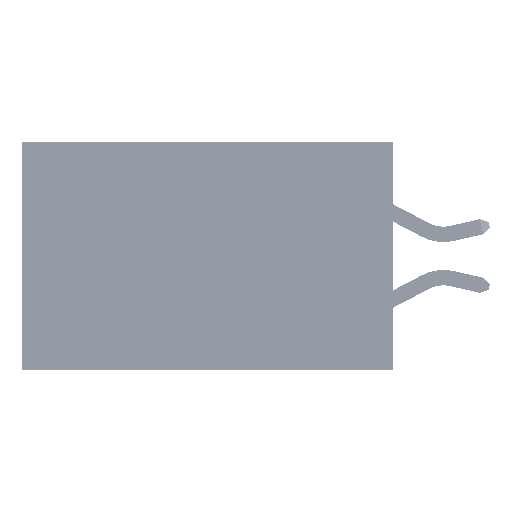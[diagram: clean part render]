
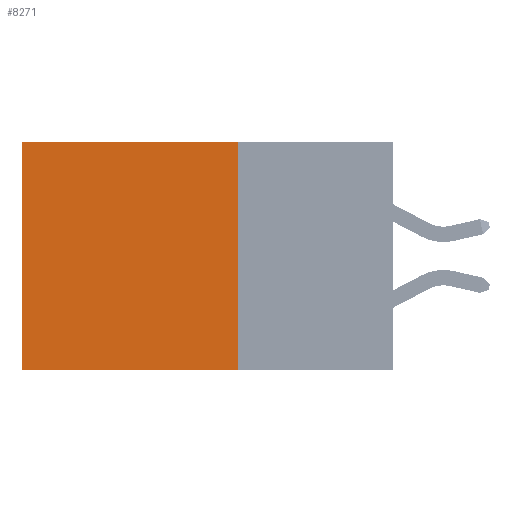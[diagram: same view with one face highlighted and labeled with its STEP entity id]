
A CAD part, left-side view. The second image highlights one B-rep face of the part: STEP entity #8271.
In plain terms, the highlighted planar face has unit normal (-1, 0, 0).
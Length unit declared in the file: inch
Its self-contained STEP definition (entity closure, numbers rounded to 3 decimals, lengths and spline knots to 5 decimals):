
#4088 = ORIENTED_EDGE ( 'NONE', *, *, #41959, .T. ) ;
#5330 = DIRECTION ( 'NONE',  ( 0., 0., -1. ) ) ;
#6642 = VERTEX_POINT ( 'NONE', #31578 ) ;
#7304 = EDGE_CURVE ( 'NONE', #40999, #11970, #41445, .T. ) ;
#7550 = VERTEX_POINT ( 'NONE', #17372 ) ;
#8271 = ADVANCED_FACE ( 'NONE', ( #8358 ), #14238, .F. ) ;
#8358 = FACE_OUTER_BOUND ( 'NONE', #43609, .T. ) ;
#9850 = ORIENTED_EDGE ( 'NONE', *, *, #7304, .F. ) ;
#10238 = VECTOR ( 'NONE', #19641, 39.37008 ) ;
#11970 = VERTEX_POINT ( 'NONE', #46373 ) ;
#13029 = CARTESIAN_POINT ( 'NONE',  ( 0.2875, 0.25, 0. ) ) ;
#14238 = PLANE ( 'NONE',  #30869 ) ;
#15359 = LINE ( 'NONE', #13029, #45191 ) ;
#15538 = ORIENTED_EDGE ( 'NONE', *, *, #29421, .F. ) ;
#17032 = CARTESIAN_POINT ( 'NONE',  ( 0.2875, 0.6, 0. ) ) ;
#17106 = CARTESIAN_POINT ( 'NONE',  ( 0.2875, 0.25, 0. ) ) ;
#17198 = DIRECTION ( 'NONE',  ( 0., 0., -1. ) ) ;
#17372 = CARTESIAN_POINT ( 'NONE',  ( 0.2875, 0.6, 0. ) ) ;
#19641 = DIRECTION ( 'NONE',  ( 0., 1., 0. ) ) ;
#22178 = DIRECTION ( 'NONE',  ( 0., 0., -1. ) ) ;
#23303 = LINE ( 'NONE', #17106, #33692 ) ;
#29421 = EDGE_CURVE ( 'NONE', #6642, #40999, #23303, .T. ) ;
#30042 = CARTESIAN_POINT ( 'NONE',  ( 0.2875, 0.25, -0.37 ) ) ;
#30869 = AXIS2_PLACEMENT_3D ( 'NONE', #41533, #45399, #22178 ) ;
#31578 = CARTESIAN_POINT ( 'NONE',  ( 0.2875, 0.25, 0. ) ) ;
#33692 = VECTOR ( 'NONE', #5330, 39.37008 ) ;
#35247 = CARTESIAN_POINT ( 'NONE',  ( 0.2875, 0.25, -0.37 ) ) ;
#36530 = DIRECTION ( 'NONE',  ( 0., 1., 0. ) ) ;
#38523 = EDGE_CURVE ( 'NONE', #7550, #11970, #49994, .T. ) ;
#39819 = VECTOR ( 'NONE', #17198, 39.37008 ) ;
#40999 = VERTEX_POINT ( 'NONE', #30042 ) ;
#41445 = LINE ( 'NONE', #35247, #10238 ) ;
#41533 = CARTESIAN_POINT ( 'NONE',  ( 0.2875, 0.25, 0. ) ) ;
#41959 = EDGE_CURVE ( 'NONE', #6642, #7550, #15359, .T. ) ;
#43595 = ORIENTED_EDGE ( 'NONE', *, *, #38523, .T. ) ;
#43609 = EDGE_LOOP ( 'NONE', ( #43595, #9850, #15538, #4088 ) ) ;
#45191 = VECTOR ( 'NONE', #36530, 39.37008 ) ;
#45399 = DIRECTION ( 'NONE',  ( 1., 0., 0. ) ) ;
#46373 = CARTESIAN_POINT ( 'NONE',  ( 0.2875, 0.6, -0.37 ) ) ;
#49994 = LINE ( 'NONE', #17032, #39819 ) ;
